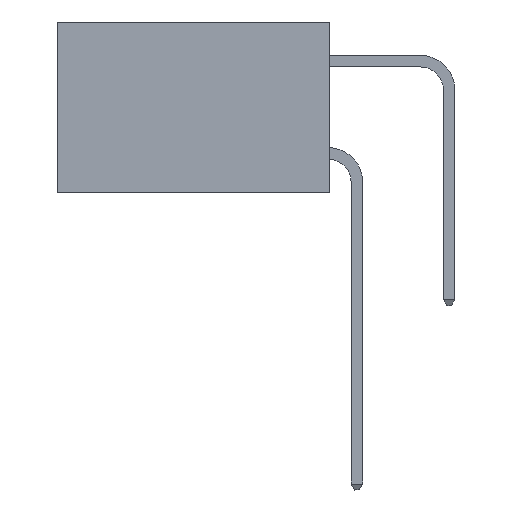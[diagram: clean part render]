
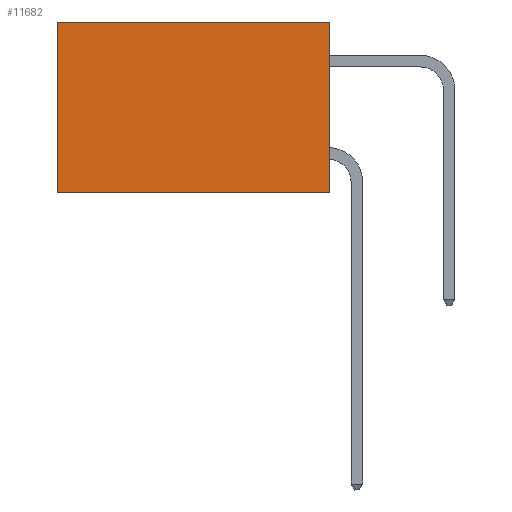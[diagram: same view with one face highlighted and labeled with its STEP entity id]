
A CAD part, left-side view. The second image highlights one B-rep face of the part: STEP entity #11682.
In plain terms, the highlighted planar face has unit normal (-1, 0, 0).
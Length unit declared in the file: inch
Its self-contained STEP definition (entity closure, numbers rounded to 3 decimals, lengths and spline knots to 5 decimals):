
#1335 = DIRECTION ( 'NONE',  ( 0., 0., -1. ) ) ;
#1368 = VERTEX_POINT ( 'NONE', #14343 ) ;
#2899 = VERTEX_POINT ( 'NONE', #24805 ) ;
#3286 = AXIS2_PLACEMENT_3D ( 'NONE', #13404, #15777, #1335 ) ;
#3904 = DIRECTION ( 'NONE',  ( 0., 1., 0. ) ) ;
#4319 = CARTESIAN_POINT ( 'NONE',  ( 0.277, 0., -0.37 ) ) ;
#6270 = LINE ( 'NONE', #21314, #11936 ) ;
#6359 = CARTESIAN_POINT ( 'NONE',  ( 0.277, 0., -0.37 ) ) ;
#7223 = EDGE_CURVE ( 'NONE', #1368, #2899, #29040, .T. ) ;
#9645 = EDGE_LOOP ( 'NONE', ( #22278, #22879, #24509, #24793 ) ) ;
#9709 = VECTOR ( 'NONE', #3904, 39.37008 ) ;
#9892 = VECTOR ( 'NONE', #25686, 39.37008 ) ;
#10032 = VECTOR ( 'NONE', #30178, 39.37008 ) ;
#10472 = LINE ( 'NONE', #6359, #9709 ) ;
#10962 = PLANE ( 'NONE',  #3286 ) ;
#11682 = ADVANCED_FACE ( 'NONE', ( #18314 ), #10962, .F. ) ;
#11936 = VECTOR ( 'NONE', #30758, 39.37008 ) ;
#12918 = CARTESIAN_POINT ( 'NONE',  ( 0.277, 0.59, -0.37 ) ) ;
#13404 = CARTESIAN_POINT ( 'NONE',  ( 0.277, 0., -0.37 ) ) ;
#14343 = CARTESIAN_POINT ( 'NONE',  ( 0.277, 0., 0. ) ) ;
#15777 = DIRECTION ( 'NONE',  ( 1., 0., 0. ) ) ;
#16033 = EDGE_CURVE ( 'NONE', #1368, #22313, #16268, .T. ) ;
#16095 = CARTESIAN_POINT ( 'NONE',  ( 0.277, 0., -0.37 ) ) ;
#16268 = LINE ( 'NONE', #16095, #9892 ) ;
#18314 = FACE_OUTER_BOUND ( 'NONE', #9645, .T. ) ;
#21314 = CARTESIAN_POINT ( 'NONE',  ( 0.277, 0.59, -0.37 ) ) ;
#22202 = EDGE_CURVE ( 'NONE', #22313, #30690, #10472, .T. ) ;
#22278 = ORIENTED_EDGE ( 'NONE', *, *, #23021, .T. ) ;
#22313 = VERTEX_POINT ( 'NONE', #4319 ) ;
#22879 = ORIENTED_EDGE ( 'NONE', *, *, #22202, .F. ) ;
#23021 = EDGE_CURVE ( 'NONE', #2899, #30690, #6270, .T. ) ;
#24509 = ORIENTED_EDGE ( 'NONE', *, *, #16033, .F. ) ;
#24793 = ORIENTED_EDGE ( 'NONE', *, *, #7223, .T. ) ;
#24805 = CARTESIAN_POINT ( 'NONE',  ( 0.277, 0.59, 0. ) ) ;
#25686 = DIRECTION ( 'NONE',  ( 0., 0., -1. ) ) ;
#29040 = LINE ( 'NONE', #30246, #10032 ) ;
#30178 = DIRECTION ( 'NONE',  ( 0., 1., 0. ) ) ;
#30246 = CARTESIAN_POINT ( 'NONE',  ( 0.277, 0., 0. ) ) ;
#30690 = VERTEX_POINT ( 'NONE', #12918 ) ;
#30758 = DIRECTION ( 'NONE',  ( 0., 0., -1. ) ) ;
